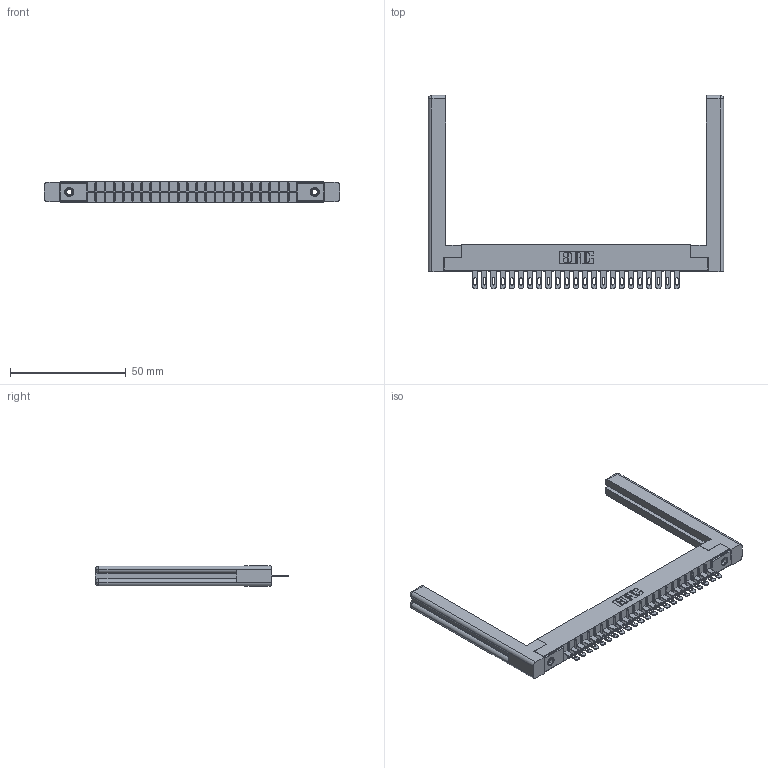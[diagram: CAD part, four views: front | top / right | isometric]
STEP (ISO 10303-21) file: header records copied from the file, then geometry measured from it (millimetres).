
FILE_DESCRIPTION (( 'STEP AP203' ), '1' );
FILE_NAME ('306-023-400-158.STEP', '2020-09-21T21:40:50', ( '' ), ( '' ), 'SwSTEP 2.0', 'SolidWorks 2020', '' );
FILE_SCHEMA (( 'CONFIG_CONTROL_DESIGN' ));
Length unit declared in the file: inch
Products named in the file (5): 306-290-001_100; 345-250-001_345-250-001-102; 306-023-400-158; 307-220-058; 306 Part_.156 Dia
Assembly tree (28 placements, depth 2):
  306-023-400-158
    306 Part_.156 Dia
    306-290-001_100  x23
    345-250-001_345-250-001-102  x2
    307-220-058  x2
Bounding box: 127.76 x 83.52 x 8.71 mm (x, y, z)
Volume: 16458.3 mm3; surface area: 18726.6 mm2
Topology: 28 solids, 28 shells, 2006 faces, 5615 edges, 3606 vertices
Faces by surface type: plane 1302, cylinder 588, sphere 92, cone 12, torus 12
Entity records: 26707 total; most frequent: CARTESIAN_POINT 4491, ORIENTED_EDGE 4392, DIRECTION 4386, EDGE_CURVE 2196, VECTOR 1700, LINE 1700, VERTEX_POINT 1394, AXIS2_PLACEMENT_3D 1343
